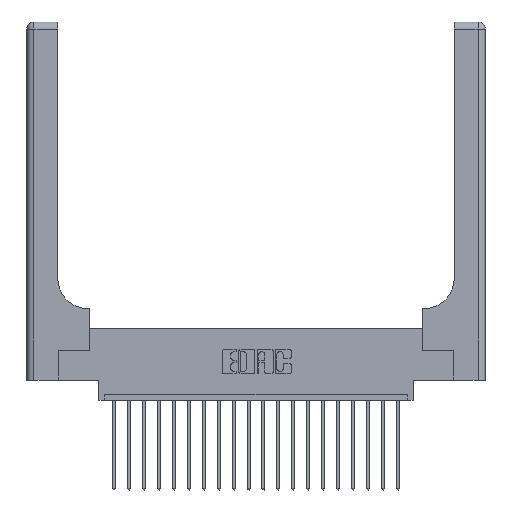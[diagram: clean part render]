
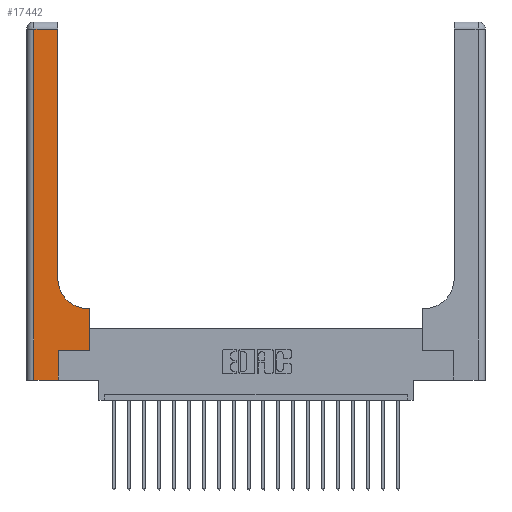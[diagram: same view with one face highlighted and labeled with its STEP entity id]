
A CAD part, top view. The second image highlights one B-rep face of the part: STEP entity #17442.
In plain terms, the highlighted planar face has unit normal (0, 0, 1).
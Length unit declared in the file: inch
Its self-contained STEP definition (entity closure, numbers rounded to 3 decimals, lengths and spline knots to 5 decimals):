
#192 = EDGE_CURVE ( 'NONE', #4473, #10117, #6136, .T. ) ;
#310 = CARTESIAN_POINT ( 'NONE',  ( 0.06, 3., 0.37 ) ) ;
#316 = LINE ( 'NONE', #11849, #7033 ) ;
#774 = DIRECTION ( 'NONE',  ( -1., 0., 0. ) ) ;
#798 = CARTESIAN_POINT ( 'NONE',  ( 0.26, 3., 0.37 ) ) ;
#1100 = EDGE_CURVE ( 'NONE', #10117, #7861, #10419, .T. ) ;
#1899 = DIRECTION ( 'NONE',  ( -1., 0., 0. ) ) ;
#1956 = VERTEX_POINT ( 'NONE', #19877 ) ;
#2020 = EDGE_CURVE ( 'NONE', #4229, #14259, #316, .T. ) ;
#2527 = EDGE_CURVE ( 'NONE', #14259, #1956, #7131, .T. ) ;
#2572 = VECTOR ( 'NONE', #4479, 39.37008 ) ;
#2915 = CARTESIAN_POINT ( 'NONE',  ( 0.51, 0.6, 0.37 ) ) ;
#3521 = CARTESIAN_POINT ( 'NONE',  ( 0., 3., 0.37 ) ) ;
#3579 = ORIENTED_EDGE ( 'NONE', *, *, #4375, .T. ) ;
#3634 = ORIENTED_EDGE ( 'NONE', *, *, #192, .T. ) ;
#3749 = LINE ( 'NONE', #310, #19288 ) ;
#3937 = FACE_OUTER_BOUND ( 'NONE', #10255, .T. ) ;
#4062 = ORIENTED_EDGE ( 'NONE', *, *, #1100, .T. ) ;
#4079 = VERTEX_POINT ( 'NONE', #14619 ) ;
#4229 = VERTEX_POINT ( 'NONE', #10323 ) ;
#4305 = VECTOR ( 'NONE', #19820, 39.37008 ) ;
#4375 = EDGE_CURVE ( 'NONE', #7861, #20048, #7225, .T. ) ;
#4381 = VECTOR ( 'NONE', #14060, 39.37008 ) ;
#4473 = VERTEX_POINT ( 'NONE', #20798 ) ;
#4479 = DIRECTION ( 'NONE',  ( 1., 0., 0. ) ) ;
#4582 = CARTESIAN_POINT ( 'NONE',  ( 0., 2.94, 0.37 ) ) ;
#5184 = DIRECTION ( 'NONE',  ( 1., 0., 0. ) ) ;
#5537 = VECTOR ( 'NONE', #6193, 39.37008 ) ;
#5665 = CARTESIAN_POINT ( 'NONE',  ( 0.06, 2.94, 0.37 ) ) ;
#6136 = LINE ( 'NONE', #10825, #18018 ) ;
#6193 = DIRECTION ( 'NONE',  ( -1., 0., 0. ) ) ;
#6829 = DIRECTION ( 'NONE',  ( 0., -1., 0. ) ) ;
#6835 = DIRECTION ( 'NONE',  ( 0., 1., 0. ) ) ;
#6920 = PLANE ( 'NONE',  #19889 ) ;
#7033 = VECTOR ( 'NONE', #6835, 39.37008 ) ;
#7131 = LINE ( 'NONE', #17156, #20732 ) ;
#7225 = LINE ( 'NONE', #798, #4381 ) ;
#7861 = VERTEX_POINT ( 'NONE', #20484 ) ;
#7882 = LINE ( 'NONE', #4582, #5537 ) ;
#8151 = EDGE_CURVE ( 'NONE', #1956, #4473, #8590, .T. ) ;
#8590 = LINE ( 'NONE', #11681, #4305 ) ;
#9006 = ORIENTED_EDGE ( 'NONE', *, *, #2020, .T. ) ;
#9499 = CARTESIAN_POINT ( 'NONE',  ( 0., 0., 0.37 ) ) ;
#9585 = CARTESIAN_POINT ( 'NONE',  ( 0.265, 0.25, 0.37 ) ) ;
#10117 = VERTEX_POINT ( 'NONE', #2915 ) ;
#10255 = EDGE_LOOP ( 'NONE', ( #3579, #14464, #11062, #14431, #9006, #15383, #11054, #3634, #4062 ) ) ;
#10323 = CARTESIAN_POINT ( 'NONE',  ( 0.265, 0., 0.37 ) ) ;
#10419 = CIRCLE ( 'NONE', #19995, 0.25 ) ;
#10825 = CARTESIAN_POINT ( 'NONE',  ( 0.26, 0.6, 0.37 ) ) ;
#11054 = ORIENTED_EDGE ( 'NONE', *, *, #8151, .T. ) ;
#11062 = ORIENTED_EDGE ( 'NONE', *, *, #19660, .T. ) ;
#11681 = CARTESIAN_POINT ( 'NONE',  ( 0.528, 0.25, 0.37 ) ) ;
#11731 = VERTEX_POINT ( 'NONE', #5665 ) ;
#11849 = CARTESIAN_POINT ( 'NONE',  ( 0.265, 0., 0.37 ) ) ;
#12244 = DIRECTION ( 'NONE',  ( 1., 0., 0. ) ) ;
#13296 = DIRECTION ( 'NONE',  ( 0., 0., -1. ) ) ;
#14060 = DIRECTION ( 'NONE',  ( 0., 1., 0. ) ) ;
#14259 = VERTEX_POINT ( 'NONE', #9585 ) ;
#14431 = ORIENTED_EDGE ( 'NONE', *, *, #19862, .T. ) ;
#14464 = ORIENTED_EDGE ( 'NONE', *, *, #16367, .T. ) ;
#14619 = CARTESIAN_POINT ( 'NONE',  ( 0.06, 0., 0.37 ) ) ;
#15383 = ORIENTED_EDGE ( 'NONE', *, *, #2527, .T. ) ;
#16367 = EDGE_CURVE ( 'NONE', #20048, #11731, #7882, .T. ) ;
#17156 = CARTESIAN_POINT ( 'NONE',  ( 0.265, 0.25, 0.37 ) ) ;
#17442 = ADVANCED_FACE ( 'NONE', ( #3937 ), #6920, .F. ) ;
#17990 = CARTESIAN_POINT ( 'NONE',  ( 0.51, 0.85, 0.37 ) ) ;
#18018 = VECTOR ( 'NONE', #774, 39.37008 ) ;
#19288 = VECTOR ( 'NONE', #6829, 39.37008 ) ;
#19660 = EDGE_CURVE ( 'NONE', #11731, #4079, #3749, .T. ) ;
#19820 = DIRECTION ( 'NONE',  ( 0., 1., 0. ) ) ;
#19843 = CARTESIAN_POINT ( 'NONE',  ( 0.26, 2.94, 0.37 ) ) ;
#19862 = EDGE_CURVE ( 'NONE', #4079, #4229, #20724, .T. ) ;
#19877 = CARTESIAN_POINT ( 'NONE',  ( 0.528, 0.25, 0.37 ) ) ;
#19889 = AXIS2_PLACEMENT_3D ( 'NONE', #3521, #19964, #1899 ) ;
#19964 = DIRECTION ( 'NONE',  ( 0., 0., -1. ) ) ;
#19995 = AXIS2_PLACEMENT_3D ( 'NONE', #17990, #13296, #5184 ) ;
#20048 = VERTEX_POINT ( 'NONE', #19843 ) ;
#20484 = CARTESIAN_POINT ( 'NONE',  ( 0.26, 0.85, 0.37 ) ) ;
#20724 = LINE ( 'NONE', #9499, #2572 ) ;
#20732 = VECTOR ( 'NONE', #12244, 39.37008 ) ;
#20798 = CARTESIAN_POINT ( 'NONE',  ( 0.528, 0.6, 0.37 ) ) ;
